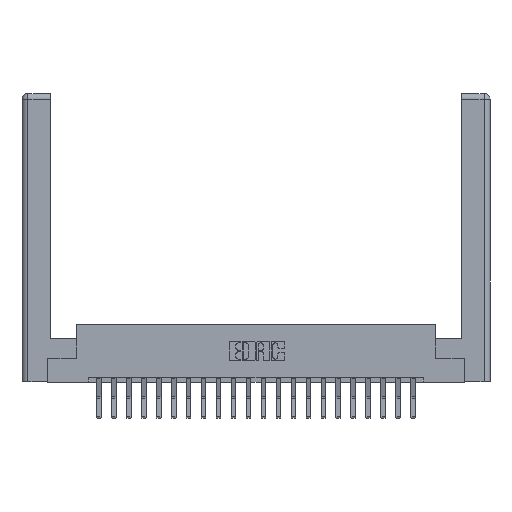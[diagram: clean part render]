
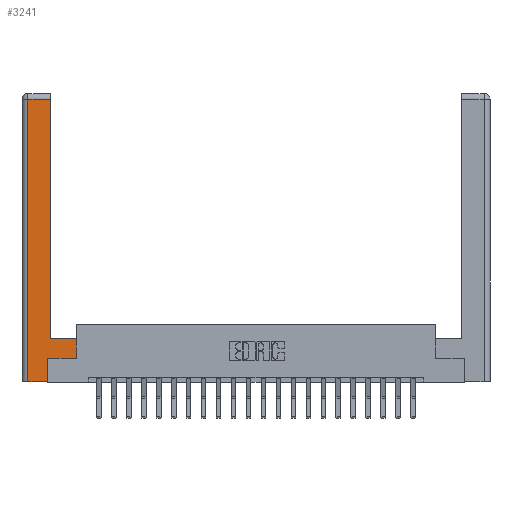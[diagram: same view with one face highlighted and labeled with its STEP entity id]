
A CAD part, top view. The second image highlights one B-rep face of the part: STEP entity #3241.
In plain terms, the highlighted planar face has unit normal (0, 0, 1).
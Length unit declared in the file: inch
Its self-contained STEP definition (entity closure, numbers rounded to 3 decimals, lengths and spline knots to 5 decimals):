
#110 = CARTESIAN_POINT ( 'NONE',  ( 0.565, 0.45, 0. ) ) ;
#318 = CARTESIAN_POINT ( 'NONE',  ( 0.0615, 2.94, 0. ) ) ;
#911 = DIRECTION ( 'NONE',  ( 0., 0., -1. ) ) ;
#1263 = EDGE_LOOP ( 'NONE', ( #17944, #5015, #19730, #2023, #16839, #2723, #15684, #12230 ) ) ;
#1308 = VERTEX_POINT ( 'NONE', #15318 ) ;
#1479 = EDGE_CURVE ( 'NONE', #15514, #6917, #14731, .T. ) ;
#1519 = LINE ( 'NONE', #21443, #3408 ) ;
#1552 = EDGE_CURVE ( 'NONE', #13370, #8461, #1519, .T. ) ;
#2023 = ORIENTED_EDGE ( 'NONE', *, *, #19768, .T. ) ;
#2034 = CARTESIAN_POINT ( 'NONE',  ( 0.0615, 0., 0. ) ) ;
#2068 = LINE ( 'NONE', #2575, #9586 ) ;
#2499 = CARTESIAN_POINT ( 'NONE',  ( 0.265, 0., 0. ) ) ;
#2549 = DIRECTION ( 'NONE',  ( -1., 0., 0. ) ) ;
#2575 = CARTESIAN_POINT ( 'NONE',  ( 0.295, 3., 0. ) ) ;
#2723 = ORIENTED_EDGE ( 'NONE', *, *, #6192, .T. ) ;
#3221 = VERTEX_POINT ( 'NONE', #19840 ) ;
#3241 = ADVANCED_FACE ( 'NONE', ( #21142 ), #14610, .F. ) ;
#3408 = VECTOR ( 'NONE', #2549, 39.37008 ) ;
#3904 = AXIS2_PLACEMENT_3D ( 'NONE', #21448, #911, #5956 ) ;
#5015 = ORIENTED_EDGE ( 'NONE', *, *, #5590, .T. ) ;
#5177 = LINE ( 'NONE', #20249, #9711 ) ;
#5590 = EDGE_CURVE ( 'NONE', #1308, #15514, #10466, .T. ) ;
#5956 = DIRECTION ( 'NONE',  ( -1., 0., 0. ) ) ;
#6192 = EDGE_CURVE ( 'NONE', #13500, #3221, #5177, .T. ) ;
#6470 = LINE ( 'NONE', #2499, #11535 ) ;
#6917 = VERTEX_POINT ( 'NONE', #21007 ) ;
#7441 = DIRECTION ( 'NONE',  ( 0., -1., 0. ) ) ;
#8461 = VERTEX_POINT ( 'NONE', #19427 ) ;
#9135 = EDGE_CURVE ( 'NONE', #8461, #1308, #2068, .T. ) ;
#9586 = VECTOR ( 'NONE', #19859, 39.37008 ) ;
#9711 = VECTOR ( 'NONE', #16708, 39.37008 ) ;
#10366 = VECTOR ( 'NONE', #7441, 39.37008 ) ;
#10466 = LINE ( 'NONE', #15608, #13469 ) ;
#11535 = VECTOR ( 'NONE', #21787, 39.37008 ) ;
#11759 = EDGE_CURVE ( 'NONE', #3221, #13370, #21406, .T. ) ;
#12230 = ORIENTED_EDGE ( 'NONE', *, *, #1552, .T. ) ;
#12540 = DIRECTION ( 'NONE',  ( 0., 1., 0. ) ) ;
#13370 = VERTEX_POINT ( 'NONE', #110 ) ;
#13469 = VECTOR ( 'NONE', #20002, 39.37008 ) ;
#13500 = VERTEX_POINT ( 'NONE', #17377 ) ;
#14610 = PLANE ( 'NONE',  #3904 ) ;
#14731 = LINE ( 'NONE', #2034, #10366 ) ;
#15318 = CARTESIAN_POINT ( 'NONE',  ( 0.295, 2.94, 0. ) ) ;
#15514 = VERTEX_POINT ( 'NONE', #318 ) ;
#15608 = CARTESIAN_POINT ( 'NONE',  ( 0.0615, 2.94, 0. ) ) ;
#15684 = ORIENTED_EDGE ( 'NONE', *, *, #11759, .T. ) ;
#16692 = CARTESIAN_POINT ( 'NONE',  ( 0.265, 0., 0. ) ) ;
#16708 = DIRECTION ( 'NONE',  ( 1., 0., 0. ) ) ;
#16839 = ORIENTED_EDGE ( 'NONE', *, *, #18450, .T. ) ;
#17042 = CARTESIAN_POINT ( 'NONE',  ( 0.265, 0.245, 0. ) ) ;
#17212 = VECTOR ( 'NONE', #20719, 39.37008 ) ;
#17377 = CARTESIAN_POINT ( 'NONE',  ( 0.265, 0.245, 0. ) ) ;
#17426 = CARTESIAN_POINT ( 'NONE',  ( 0.565, 0.45, 0. ) ) ;
#17944 = ORIENTED_EDGE ( 'NONE', *, *, #9135, .T. ) ;
#18450 = EDGE_CURVE ( 'NONE', #21976, #13500, #21876, .T. ) ;
#19427 = CARTESIAN_POINT ( 'NONE',  ( 0.295, 0.45, 0. ) ) ;
#19730 = ORIENTED_EDGE ( 'NONE', *, *, #1479, .T. ) ;
#19768 = EDGE_CURVE ( 'NONE', #6917, #21976, #6470, .T. ) ;
#19840 = CARTESIAN_POINT ( 'NONE',  ( 0.565, 0.245, 0. ) ) ;
#19859 = DIRECTION ( 'NONE',  ( 0., 1., 0. ) ) ;
#20002 = DIRECTION ( 'NONE',  ( -1., 0., 0. ) ) ;
#20249 = CARTESIAN_POINT ( 'NONE',  ( 0.565, 0.245, 0. ) ) ;
#20719 = DIRECTION ( 'NONE',  ( 0., 1., 0. ) ) ;
#21007 = CARTESIAN_POINT ( 'NONE',  ( 0.0615, 0., 0. ) ) ;
#21142 = FACE_OUTER_BOUND ( 'NONE', #1263, .T. ) ;
#21406 = LINE ( 'NONE', #17426, #21998 ) ;
#21443 = CARTESIAN_POINT ( 'NONE',  ( 0.295, 0.45, 0. ) ) ;
#21448 = CARTESIAN_POINT ( 'NONE',  ( 0., 0., 0. ) ) ;
#21787 = DIRECTION ( 'NONE',  ( 1., 0., 0. ) ) ;
#21876 = LINE ( 'NONE', #17042, #17212 ) ;
#21976 = VERTEX_POINT ( 'NONE', #16692 ) ;
#21998 = VECTOR ( 'NONE', #12540, 39.37008 ) ;
